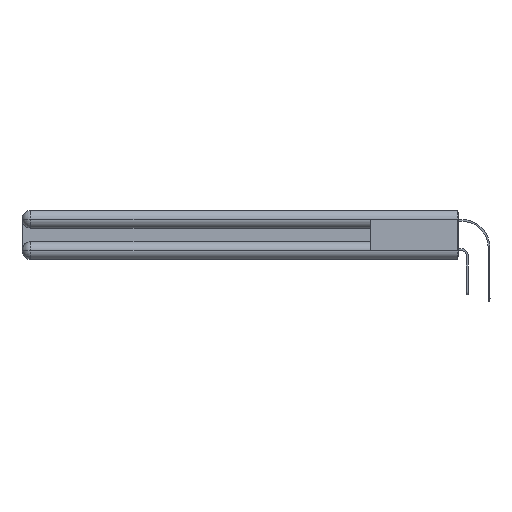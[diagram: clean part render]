
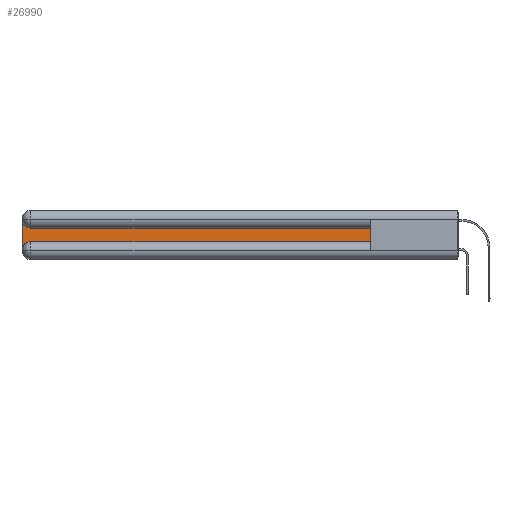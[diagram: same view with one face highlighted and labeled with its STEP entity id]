
A CAD part, left-side view. The second image highlights one B-rep face of the part: STEP entity #26990.
In plain terms, the highlighted planar face has unit normal (-1, 0, 0).
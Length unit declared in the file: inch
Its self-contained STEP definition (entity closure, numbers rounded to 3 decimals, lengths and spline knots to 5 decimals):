
#82 = CARTESIAN_POINT ( 'NONE',  ( 0.075, 0.6, -0.2175 ) ) ;
#544 = ORIENTED_EDGE ( 'NONE', *, *, #6562, .T. ) ;
#1350 = CARTESIAN_POINT ( 'NONE',  ( 0.075, 2.94, -0.2175 ) ) ;
#2261 = CARTESIAN_POINT ( 'NONE',  ( 0.075, 3., -0.2775 ) ) ;
#2500 = EDGE_CURVE ( 'NONE', #22902, #3749, #23913, .T. ) ;
#2914 = EDGE_LOOP ( 'NONE', ( #18331, #2992, #544, #13867, #17025, #20250 ) ) ;
#2992 = ORIENTED_EDGE ( 'NONE', *, *, #2500, .T. ) ;
#3287 = LINE ( 'NONE', #14642, #11690 ) ;
#3641 = VERTEX_POINT ( 'NONE', #25963 ) ;
#3749 = VERTEX_POINT ( 'NONE', #10171 ) ;
#5535 = CARTESIAN_POINT ( 'NONE',  ( 0.075, 2.94, -0.1225 ) ) ;
#5652 = DIRECTION ( 'NONE',  ( 1., 0., 0. ) ) ;
#5871 = DIRECTION ( 'NONE',  ( 0., 0., -1. ) ) ;
#6317 = DIRECTION ( 'NONE',  ( 1., 0., 0. ) ) ;
#6562 = EDGE_CURVE ( 'NONE', #3749, #11961, #3287, .T. ) ;
#6668 = AXIS2_PLACEMENT_3D ( 'NONE', #12449, #5652, #28562 ) ;
#7496 = DIRECTION ( 'NONE',  ( 0., 1., 0. ) ) ;
#7774 = PLANE ( 'NONE',  #6668 ) ;
#7982 = EDGE_CURVE ( 'NONE', #11961, #15009, #14253, .T. ) ;
#8433 = CARTESIAN_POINT ( 'NONE',  ( 0.075, 2.94, -0.2775 ) ) ;
#8924 = AXIS2_PLACEMENT_3D ( 'NONE', #8433, #6317, #5871 ) ;
#9109 = LINE ( 'NONE', #11524, #13733 ) ;
#9199 = EDGE_CURVE ( 'NONE', #3641, #26343, #16752, .T. ) ;
#10171 = CARTESIAN_POINT ( 'NONE',  ( 0.075, 3., -0.0625 ) ) ;
#11156 = CARTESIAN_POINT ( 'NONE',  ( 0.075, 0.6, -0.1225 ) ) ;
#11524 = CARTESIAN_POINT ( 'NONE',  ( 0.075, 0.6, -0.2175 ) ) ;
#11690 = VECTOR ( 'NONE', #24085, 39.37008 ) ;
#11961 = VERTEX_POINT ( 'NONE', #2261 ) ;
#12267 = DIRECTION ( 'NONE',  ( 1., 0., 0. ) ) ;
#12449 = CARTESIAN_POINT ( 'NONE',  ( 0.075, 3., -0.1225 ) ) ;
#13733 = VECTOR ( 'NONE', #22917, 39.37008 ) ;
#13867 = ORIENTED_EDGE ( 'NONE', *, *, #7982, .T. ) ;
#14253 = CIRCLE ( 'NONE', #8924, 0.06 ) ;
#14642 = CARTESIAN_POINT ( 'NONE',  ( 0.075, 3., -0.2175 ) ) ;
#15009 = VERTEX_POINT ( 'NONE', #1350 ) ;
#15202 = VECTOR ( 'NONE', #7496, 39.37008 ) ;
#16750 = EDGE_CURVE ( 'NONE', #26343, #22902, #26601, .T. ) ;
#16752 = LINE ( 'NONE', #82, #28287 ) ;
#17025 = ORIENTED_EDGE ( 'NONE', *, *, #17545, .T. ) ;
#17545 = EDGE_CURVE ( 'NONE', #15009, #3641, #9109, .T. ) ;
#18331 = ORIENTED_EDGE ( 'NONE', *, *, #16750, .T. ) ;
#20250 = ORIENTED_EDGE ( 'NONE', *, *, #9199, .T. ) ;
#22461 = AXIS2_PLACEMENT_3D ( 'NONE', #28980, #12267, #23828 ) ;
#22902 = VERTEX_POINT ( 'NONE', #5535 ) ;
#22917 = DIRECTION ( 'NONE',  ( 0., -1., 0. ) ) ;
#23828 = DIRECTION ( 'NONE',  ( 0., 0., -1. ) ) ;
#23868 = CARTESIAN_POINT ( 'NONE',  ( 0.075, 0.6, -0.1225 ) ) ;
#23913 = CIRCLE ( 'NONE', #22461, 0.06 ) ;
#24085 = DIRECTION ( 'NONE',  ( 0., 0., -1. ) ) ;
#25855 = DIRECTION ( 'NONE',  ( 0., 0., 1. ) ) ;
#25963 = CARTESIAN_POINT ( 'NONE',  ( 0.075, 0.6, -0.2175 ) ) ;
#26343 = VERTEX_POINT ( 'NONE', #11156 ) ;
#26601 = LINE ( 'NONE', #23868, #15202 ) ;
#26990 = ADVANCED_FACE ( 'NONE', ( #28701 ), #7774, .F. ) ;
#28287 = VECTOR ( 'NONE', #25855, 39.37008 ) ;
#28562 = DIRECTION ( 'NONE',  ( 0., 0., -1. ) ) ;
#28701 = FACE_OUTER_BOUND ( 'NONE', #2914, .T. ) ;
#28980 = CARTESIAN_POINT ( 'NONE',  ( 0.075, 2.94, -0.0625 ) ) ;
